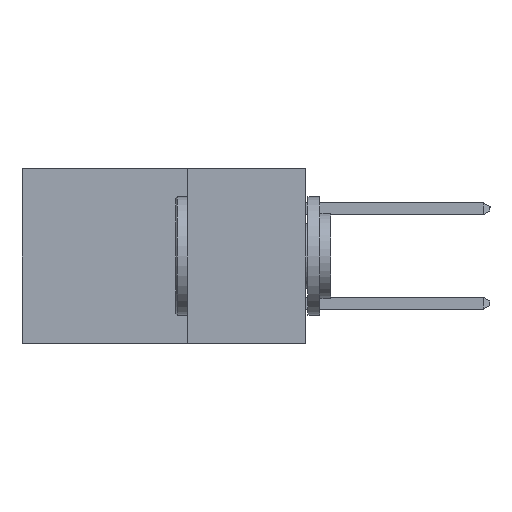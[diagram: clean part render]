
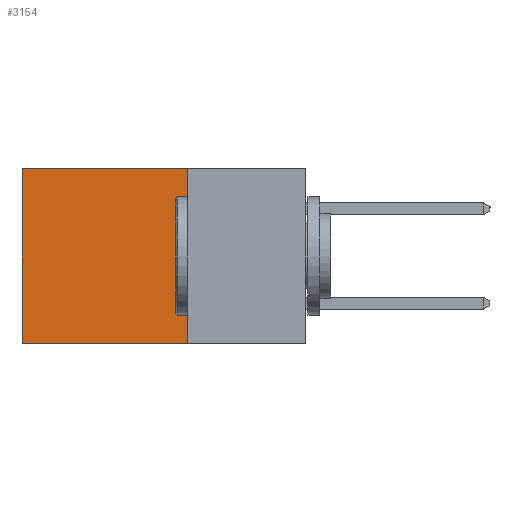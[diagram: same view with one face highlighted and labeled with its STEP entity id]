
A CAD part, left-side view. The second image highlights one B-rep face of the part: STEP entity #3154.
In plain terms, the highlighted planar face has unit normal (-1, 0, 0).
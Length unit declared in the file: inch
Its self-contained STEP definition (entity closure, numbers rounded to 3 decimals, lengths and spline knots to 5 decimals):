
#182 = DIRECTION ( 'NONE',  ( 0., 0., -1. ) ) ;
#1849 = VERTEX_POINT ( 'NONE', #3066 ) ;
#3066 = CARTESIAN_POINT ( 'NONE',  ( 0.2615, 0.25, -0.37 ) ) ;
#3154 = ADVANCED_FACE ( 'NONE', ( #12265 ), #14054, .F. ) ;
#3507 = VERTEX_POINT ( 'NONE', #11427 ) ;
#3831 = LINE ( 'NONE', #4266, #20853 ) ;
#4175 = CARTESIAN_POINT ( 'NONE',  ( 0.2615, 0.6, -0.37 ) ) ;
#4266 = CARTESIAN_POINT ( 'NONE',  ( 0.2615, 0.25, -0.37 ) ) ;
#4659 = EDGE_CURVE ( 'NONE', #3507, #7660, #5645, .T. ) ;
#5035 = AXIS2_PLACEMENT_3D ( 'NONE', #20881, #12371, #19193 ) ;
#5645 = LINE ( 'NONE', #15465, #10416 ) ;
#5849 = DIRECTION ( 'NONE',  ( 0., 1., 0. ) ) ;
#7660 = VERTEX_POINT ( 'NONE', #4175 ) ;
#8341 = CARTESIAN_POINT ( 'NONE',  ( 0.2615, 0.25, -0.37 ) ) ;
#8550 = DIRECTION ( 'NONE',  ( 0., 0., -1. ) ) ;
#10416 = VECTOR ( 'NONE', #182, 39.37008 ) ;
#10844 = DIRECTION ( 'NONE',  ( 0., 1., 0. ) ) ;
#11348 = ORIENTED_EDGE ( 'NONE', *, *, #11827, .F. ) ;
#11427 = CARTESIAN_POINT ( 'NONE',  ( 0.2615, 0.6, 0. ) ) ;
#11827 = EDGE_CURVE ( 'NONE', #16244, #1849, #21752, .T. ) ;
#12167 = CARTESIAN_POINT ( 'NONE',  ( 0.2615, 0.25, 0. ) ) ;
#12265 = FACE_OUTER_BOUND ( 'NONE', #13168, .T. ) ;
#12371 = DIRECTION ( 'NONE',  ( 1., 0., 0. ) ) ;
#12421 = LINE ( 'NONE', #12866, #15394 ) ;
#12866 = CARTESIAN_POINT ( 'NONE',  ( 0.2615, 0.25, 0. ) ) ;
#13168 = EDGE_LOOP ( 'NONE', ( #16757, #13717, #11348, #16119 ) ) ;
#13717 = ORIENTED_EDGE ( 'NONE', *, *, #14653, .F. ) ;
#14054 = PLANE ( 'NONE',  #5035 ) ;
#14653 = EDGE_CURVE ( 'NONE', #1849, #7660, #3831, .T. ) ;
#15394 = VECTOR ( 'NONE', #5849, 39.37008 ) ;
#15465 = CARTESIAN_POINT ( 'NONE',  ( 0.2615, 0.6, -0.37 ) ) ;
#16119 = ORIENTED_EDGE ( 'NONE', *, *, #18719, .T. ) ;
#16244 = VERTEX_POINT ( 'NONE', #12167 ) ;
#16757 = ORIENTED_EDGE ( 'NONE', *, *, #4659, .T. ) ;
#17151 = VECTOR ( 'NONE', #8550, 39.37008 ) ;
#18719 = EDGE_CURVE ( 'NONE', #16244, #3507, #12421, .T. ) ;
#19193 = DIRECTION ( 'NONE',  ( 0., 0., -1. ) ) ;
#20853 = VECTOR ( 'NONE', #10844, 39.37008 ) ;
#20881 = CARTESIAN_POINT ( 'NONE',  ( 0.2615, 0.25, -0.37 ) ) ;
#21752 = LINE ( 'NONE', #8341, #17151 ) ;
